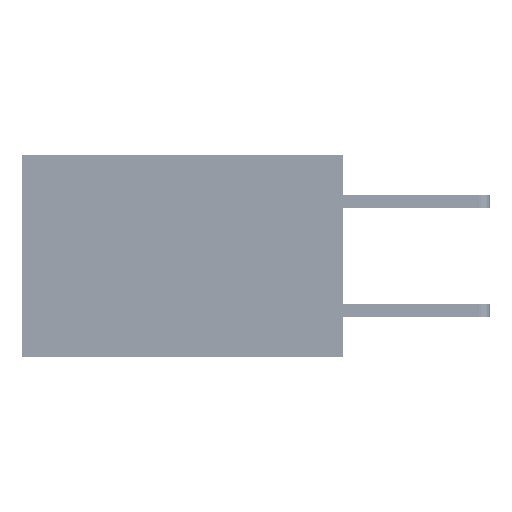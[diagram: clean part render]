
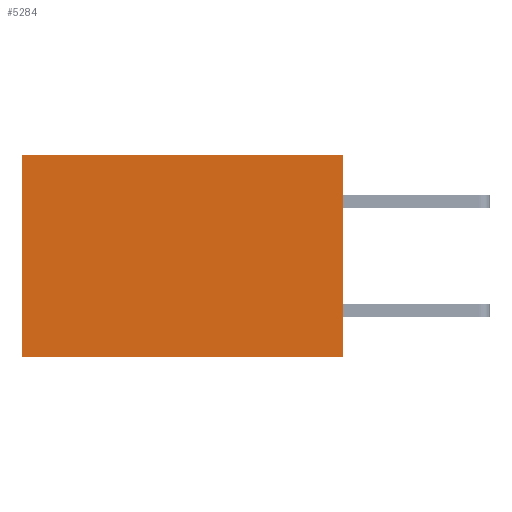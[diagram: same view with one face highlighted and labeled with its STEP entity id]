
A CAD part, left-side view. The second image highlights one B-rep face of the part: STEP entity #5284.
In plain terms, the highlighted planar face has unit normal (-1, 0, 0).
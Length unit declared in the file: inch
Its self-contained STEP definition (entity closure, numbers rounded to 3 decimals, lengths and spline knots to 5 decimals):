
#240 = DIRECTION ( 'NONE',  ( 0., 1., 0. ) ) ;
#1293 = LINE ( 'NONE', #33195, #19626 ) ;
#2286 = PLANE ( 'NONE',  #10858 ) ;
#5174 = LINE ( 'NONE', #5346, #17716 ) ;
#5284 = ADVANCED_FACE ( 'NONE', ( #26410 ), #2286, .F. ) ;
#5346 = CARTESIAN_POINT ( 'NONE',  ( 0.277, 0., -0.37 ) ) ;
#5771 = CARTESIAN_POINT ( 'NONE',  ( 0.277, 0., -0.37 ) ) ;
#7390 = DIRECTION ( 'NONE',  ( 1., 0., 0. ) ) ;
#9056 = DIRECTION ( 'NONE',  ( 0., 0., -1. ) ) ;
#10657 = VECTOR ( 'NONE', #29864, 39.37008 ) ;
#10858 = AXIS2_PLACEMENT_3D ( 'NONE', #13028, #7390, #26930 ) ;
#10989 = DIRECTION ( 'NONE',  ( 0., 1., 0. ) ) ;
#11125 = EDGE_LOOP ( 'NONE', ( #13782, #18240, #23478, #33464 ) ) ;
#13028 = CARTESIAN_POINT ( 'NONE',  ( 0.277, 0., -0.37 ) ) ;
#13752 = VECTOR ( 'NONE', #240, 39.37008 ) ;
#13782 = ORIENTED_EDGE ( 'NONE', *, *, #16191, .T. ) ;
#14348 = VERTEX_POINT ( 'NONE', #5771 ) ;
#16191 = EDGE_CURVE ( 'NONE', #26195, #25100, #32691, .T. ) ;
#17716 = VECTOR ( 'NONE', #10989, 39.37008 ) ;
#18240 = ORIENTED_EDGE ( 'NONE', *, *, #29183, .F. ) ;
#19417 = VERTEX_POINT ( 'NONE', #30759 ) ;
#19626 = VECTOR ( 'NONE', #9056, 39.37008 ) ;
#22920 = CARTESIAN_POINT ( 'NONE',  ( 0.277, 0.59, -0.37 ) ) ;
#23478 = ORIENTED_EDGE ( 'NONE', *, *, #25418, .F. ) ;
#24386 = CARTESIAN_POINT ( 'NONE',  ( 0.277, 0., 0. ) ) ;
#25100 = VERTEX_POINT ( 'NONE', #28983 ) ;
#25418 = EDGE_CURVE ( 'NONE', #19417, #14348, #1293, .T. ) ;
#26195 = VERTEX_POINT ( 'NONE', #33441 ) ;
#26410 = FACE_OUTER_BOUND ( 'NONE', #11125, .T. ) ;
#26930 = DIRECTION ( 'NONE',  ( 0., 0., -1. ) ) ;
#27037 = LINE ( 'NONE', #24386, #13752 ) ;
#28983 = CARTESIAN_POINT ( 'NONE',  ( 0.277, 0.59, -0.37 ) ) ;
#29183 = EDGE_CURVE ( 'NONE', #14348, #25100, #5174, .T. ) ;
#29864 = DIRECTION ( 'NONE',  ( 0., 0., -1. ) ) ;
#30577 = EDGE_CURVE ( 'NONE', #19417, #26195, #27037, .T. ) ;
#30759 = CARTESIAN_POINT ( 'NONE',  ( 0.277, 0., 0. ) ) ;
#32691 = LINE ( 'NONE', #22920, #10657 ) ;
#33195 = CARTESIAN_POINT ( 'NONE',  ( 0.277, 0., -0.37 ) ) ;
#33441 = CARTESIAN_POINT ( 'NONE',  ( 0.277, 0.59, 0. ) ) ;
#33464 = ORIENTED_EDGE ( 'NONE', *, *, #30577, .T. ) ;
